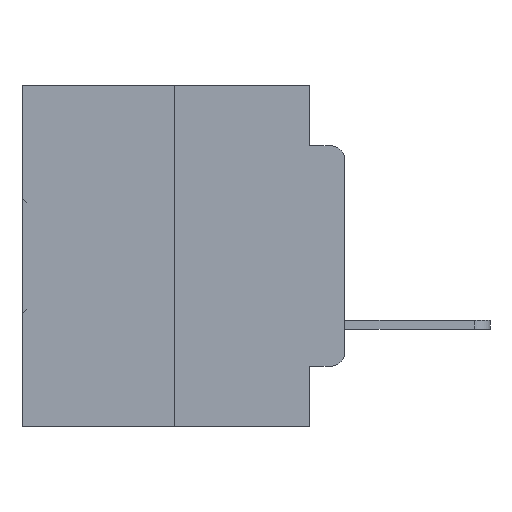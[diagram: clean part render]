
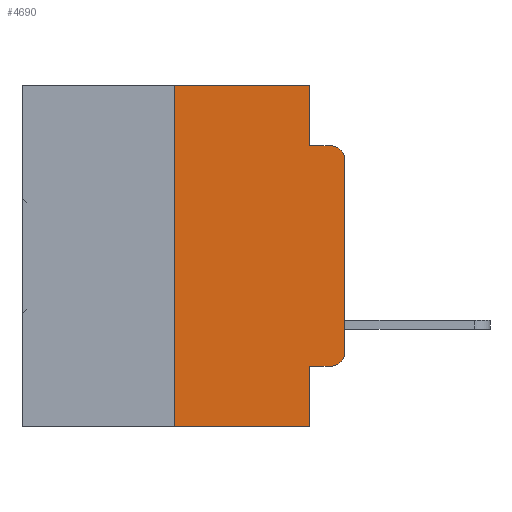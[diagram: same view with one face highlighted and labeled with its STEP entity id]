
A CAD part, left-side view. The second image highlights one B-rep face of the part: STEP entity #4690.
In plain terms, the highlighted planar face has unit normal (-1, 0, 0).
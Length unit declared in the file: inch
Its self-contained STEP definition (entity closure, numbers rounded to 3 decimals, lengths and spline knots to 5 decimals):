
#33 = VERTEX_POINT ( 'NONE', #9548 ) ;
#210 = DIRECTION ( 'NONE',  ( 0., 0., -1. ) ) ;
#586 = AXIS2_PLACEMENT_3D ( 'NONE', #10577, #27597, #13135 ) ;
#778 = VERTEX_POINT ( 'NONE', #16703 ) ;
#1641 = CARTESIAN_POINT ( 'NONE',  ( 0., 0.473, 0. ) ) ;
#2054 = LINE ( 'NONE', #16685, #14315 ) ;
#2300 = FACE_OUTER_BOUND ( 'NONE', #28868, .T. ) ;
#2827 = VERTEX_POINT ( 'NONE', #16539 ) ;
#3220 = CARTESIAN_POINT ( 'NONE',  ( 0., 0.051, -0.0885 ) ) ;
#4087 = EDGE_CURVE ( 'NONE', #5118, #20394, #4768, .T. ) ;
#4538 = CARTESIAN_POINT ( 'NONE',  ( 0., 0.25, 0. ) ) ;
#4610 = DIRECTION ( 'NONE',  ( 0., 0., -1. ) ) ;
#4690 = ADVANCED_FACE ( 'NONE', ( #2300 ), #8432, .F. ) ;
#4768 = CIRCLE ( 'NONE', #15040, 0.02 ) ;
#5103 = VERTEX_POINT ( 'NONE', #16178 ) ;
#5118 = VERTEX_POINT ( 'NONE', #14668 ) ;
#5909 = DIRECTION ( 'NONE',  ( 0., -1., 0. ) ) ;
#6143 = DIRECTION ( 'NONE',  ( 0., -1., 0. ) ) ;
#6277 = DIRECTION ( 'NONE',  ( 0., 0., -1. ) ) ;
#6377 = DIRECTION ( 'NONE',  ( 0., 0., 1. ) ) ;
#6975 = VERTEX_POINT ( 'NONE', #23819 ) ;
#7754 = EDGE_CURVE ( 'NONE', #21900, #5118, #25904, .T. ) ;
#8122 = CARTESIAN_POINT ( 'NONE',  ( 0., 0.02, -0.0885 ) ) ;
#8432 = PLANE ( 'NONE',  #13152 ) ;
#9548 = CARTESIAN_POINT ( 'NONE',  ( 0., 0.051, -0.4115 ) ) ;
#9662 = DIRECTION ( 'NONE',  ( 0., -1., 0. ) ) ;
#9732 = VECTOR ( 'NONE', #5909, 39.37008 ) ;
#10346 = VERTEX_POINT ( 'NONE', #28074 ) ;
#10577 = CARTESIAN_POINT ( 'NONE',  ( 0., 0.02, -0.3915 ) ) ;
#11025 = DIRECTION ( 'NONE',  ( 0., -1., 0. ) ) ;
#11063 = VECTOR ( 'NONE', #9662, 39.37008 ) ;
#11809 = EDGE_CURVE ( 'NONE', #2827, #21900, #26580, .T. ) ;
#12405 = CARTESIAN_POINT ( 'NONE',  ( 0., 0.02, -0.1085 ) ) ;
#12518 = DIRECTION ( 'NONE',  ( -1., 0., 0. ) ) ;
#12692 = EDGE_CURVE ( 'NONE', #10346, #6975, #25135, .T. ) ;
#13135 = DIRECTION ( 'NONE',  ( 0., 0., -1. ) ) ;
#13152 = AXIS2_PLACEMENT_3D ( 'NONE', #31924, #16179, #4610 ) ;
#14315 = VECTOR ( 'NONE', #19194, 39.37008 ) ;
#14668 = CARTESIAN_POINT ( 'NONE',  ( 0., 0., -0.1085 ) ) ;
#14825 = EDGE_CURVE ( 'NONE', #5103, #778, #30283, .T. ) ;
#14842 = CARTESIAN_POINT ( 'NONE',  ( 0., 0.051, -0.0885 ) ) ;
#15040 = AXIS2_PLACEMENT_3D ( 'NONE', #12405, #12518, #6277 ) ;
#15230 = EDGE_CURVE ( 'NONE', #33, #2827, #19766, .T. ) ;
#16178 = CARTESIAN_POINT ( 'NONE',  ( 0., 0.25, 0. ) ) ;
#16179 = DIRECTION ( 'NONE',  ( 1., 0., 0. ) ) ;
#16539 = CARTESIAN_POINT ( 'NONE',  ( 0., 0.02, -0.4115 ) ) ;
#16685 = CARTESIAN_POINT ( 'NONE',  ( 0., 0.051, 0. ) ) ;
#16703 = CARTESIAN_POINT ( 'NONE',  ( 0., 0.051, 0. ) ) ;
#17734 = LINE ( 'NONE', #4538, #24194 ) ;
#17905 = CARTESIAN_POINT ( 'NONE',  ( 0., 0., -0.3915 ) ) ;
#18612 = EDGE_CURVE ( 'NONE', #33, #6975, #31039, .T. ) ;
#18746 = VECTOR ( 'NONE', #11025, 39.37008 ) ;
#19194 = DIRECTION ( 'NONE',  ( 0., 0., -1. ) ) ;
#19766 = LINE ( 'NONE', #23797, #32076 ) ;
#19933 = DIRECTION ( 'NONE',  ( 0., 0., 1. ) ) ;
#20394 = VERTEX_POINT ( 'NONE', #8122 ) ;
#20899 = CARTESIAN_POINT ( 'NONE',  ( 0., 0.473, -0.5 ) ) ;
#21900 = VERTEX_POINT ( 'NONE', #17905 ) ;
#23489 = EDGE_CURVE ( 'NONE', #10346, #5103, #17734, .T. ) ;
#23797 = CARTESIAN_POINT ( 'NONE',  ( 0., 0.051, -0.4115 ) ) ;
#23819 = CARTESIAN_POINT ( 'NONE',  ( 0., 0.051, -0.5 ) ) ;
#23999 = CARTESIAN_POINT ( 'NONE',  ( 0., 0., 0. ) ) ;
#24194 = VECTOR ( 'NONE', #19933, 39.37008 ) ;
#24502 = VECTOR ( 'NONE', #6377, 39.37008 ) ;
#24598 = ORIENTED_EDGE ( 'NONE', *, *, #7754, .T. ) ;
#25135 = LINE ( 'NONE', #20899, #18746 ) ;
#25832 = ORIENTED_EDGE ( 'NONE', *, *, #4087, .T. ) ;
#25904 = LINE ( 'NONE', #23999, #24502 ) ;
#26337 = ORIENTED_EDGE ( 'NONE', *, *, #29568, .F. ) ;
#26425 = ORIENTED_EDGE ( 'NONE', *, *, #28029, .F. ) ;
#26580 = CIRCLE ( 'NONE', #586, 0.02 ) ;
#26710 = VERTEX_POINT ( 'NONE', #14842 ) ;
#26816 = ORIENTED_EDGE ( 'NONE', *, *, #14825, .F. ) ;
#26868 = ORIENTED_EDGE ( 'NONE', *, *, #23489, .F. ) ;
#26998 = ORIENTED_EDGE ( 'NONE', *, *, #12692, .T. ) ;
#27597 = DIRECTION ( 'NONE',  ( -1., 0., 0. ) ) ;
#28029 = EDGE_CURVE ( 'NONE', #778, #26710, #2054, .T. ) ;
#28074 = CARTESIAN_POINT ( 'NONE',  ( 0., 0.25, -0.5 ) ) ;
#28149 = ORIENTED_EDGE ( 'NONE', *, *, #18612, .F. ) ;
#28868 = EDGE_LOOP ( 'NONE', ( #24598, #25832, #26337, #26425, #26816, #26868, #26998, #28149, #29743, #29929 ) ) ;
#29069 = LINE ( 'NONE', #3220, #9732 ) ;
#29568 = EDGE_CURVE ( 'NONE', #26710, #20394, #29069, .T. ) ;
#29607 = VECTOR ( 'NONE', #210, 39.37008 ) ;
#29743 = ORIENTED_EDGE ( 'NONE', *, *, #15230, .T. ) ;
#29929 = ORIENTED_EDGE ( 'NONE', *, *, #11809, .T. ) ;
#30114 = CARTESIAN_POINT ( 'NONE',  ( 0., 0.051, 0. ) ) ;
#30283 = LINE ( 'NONE', #1641, #11063 ) ;
#31039 = LINE ( 'NONE', #30114, #29607 ) ;
#31924 = CARTESIAN_POINT ( 'NONE',  ( 0., 0.473, 0. ) ) ;
#32076 = VECTOR ( 'NONE', #6143, 39.37008 ) ;
